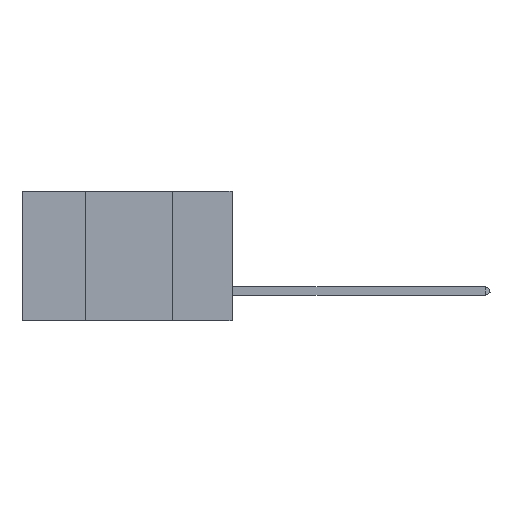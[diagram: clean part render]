
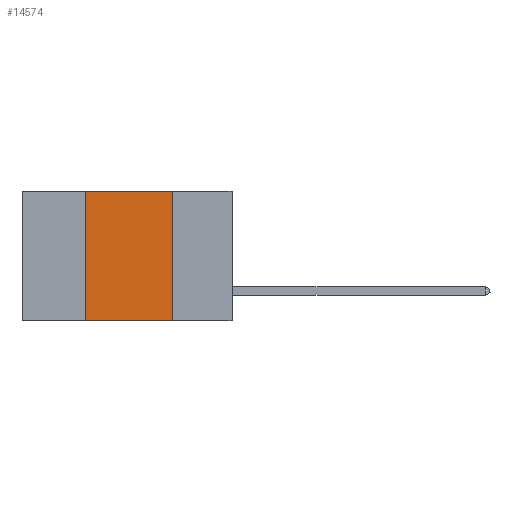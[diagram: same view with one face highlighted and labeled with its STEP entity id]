
A CAD part, left-side view. The second image highlights one B-rep face of the part: STEP entity #14574.
In plain terms, the highlighted planar face has unit normal (-1, 0, 0).
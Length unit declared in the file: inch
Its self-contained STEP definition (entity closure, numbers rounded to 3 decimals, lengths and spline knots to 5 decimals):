
#180 = ORIENTED_EDGE ( 'NONE', *, *, #1056, .F. ) ;
#491 = CARTESIAN_POINT ( 'NONE',  ( 0., 0.17, -0.37 ) ) ;
#695 = LINE ( 'NONE', #5453, #13090 ) ;
#763 = ORIENTED_EDGE ( 'NONE', *, *, #2744, .F. ) ;
#1056 = EDGE_CURVE ( 'NONE', #3967, #15156, #4562, .T. ) ;
#1243 = EDGE_CURVE ( 'NONE', #1497, #3967, #695, .T. ) ;
#1371 = CARTESIAN_POINT ( 'NONE',  ( 0., 0.17, 0. ) ) ;
#1497 = VERTEX_POINT ( 'NONE', #14977 ) ;
#1883 = AXIS2_PLACEMENT_3D ( 'NONE', #15048, #12493, #2086 ) ;
#2057 = ORIENTED_EDGE ( 'NONE', *, *, #2789, .T. ) ;
#2086 = DIRECTION ( 'NONE',  ( 0., 0., -1. ) ) ;
#2744 = EDGE_CURVE ( 'NONE', #15156, #16825, #13446, .T. ) ;
#2789 = EDGE_CURVE ( 'NONE', #1497, #16825, #3500, .T. ) ;
#3500 = LINE ( 'NONE', #4120, #14050 ) ;
#3967 = VERTEX_POINT ( 'NONE', #4044 ) ;
#4044 = CARTESIAN_POINT ( 'NONE',  ( 0., 0.42, 0. ) ) ;
#4120 = CARTESIAN_POINT ( 'NONE',  ( 0., 0.6, -0.37 ) ) ;
#4361 = CARTESIAN_POINT ( 'NONE',  ( 0., 0.17, 0. ) ) ;
#4562 = LINE ( 'NONE', #6684, #12678 ) ;
#5453 = CARTESIAN_POINT ( 'NONE',  ( 0., 0.42, 0. ) ) ;
#6684 = CARTESIAN_POINT ( 'NONE',  ( 0., 0.6, 0. ) ) ;
#8970 = FACE_OUTER_BOUND ( 'NONE', #9292, .T. ) ;
#9292 = EDGE_LOOP ( 'NONE', ( #763, #180, #11736, #2057 ) ) ;
#9453 = DIRECTION ( 'NONE',  ( 0., 0., 1. ) ) ;
#10206 = VECTOR ( 'NONE', #13081, 39.37008 ) ;
#10480 = DIRECTION ( 'NONE',  ( 0., -1., 0. ) ) ;
#11267 = PLANE ( 'NONE',  #1883 ) ;
#11736 = ORIENTED_EDGE ( 'NONE', *, *, #1243, .F. ) ;
#11905 = DIRECTION ( 'NONE',  ( 0., -1., 0. ) ) ;
#12493 = DIRECTION ( 'NONE',  ( 1., 0., 0. ) ) ;
#12678 = VECTOR ( 'NONE', #11905, 39.37008 ) ;
#13081 = DIRECTION ( 'NONE',  ( 0., 0., -1. ) ) ;
#13090 = VECTOR ( 'NONE', #9453, 39.37008 ) ;
#13446 = LINE ( 'NONE', #1371, #10206 ) ;
#14050 = VECTOR ( 'NONE', #10480, 39.37008 ) ;
#14574 = ADVANCED_FACE ( 'NONE', ( #8970 ), #11267, .F. ) ;
#14977 = CARTESIAN_POINT ( 'NONE',  ( 0., 0.42, -0.37 ) ) ;
#15048 = CARTESIAN_POINT ( 'NONE',  ( 0., 0.6, 0. ) ) ;
#15156 = VERTEX_POINT ( 'NONE', #4361 ) ;
#16825 = VERTEX_POINT ( 'NONE', #491 ) ;
